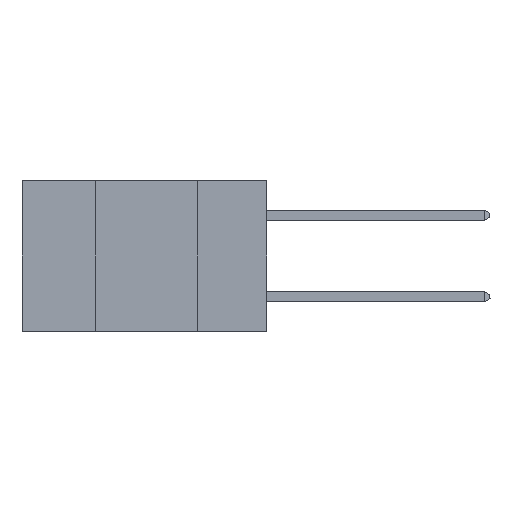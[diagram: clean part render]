
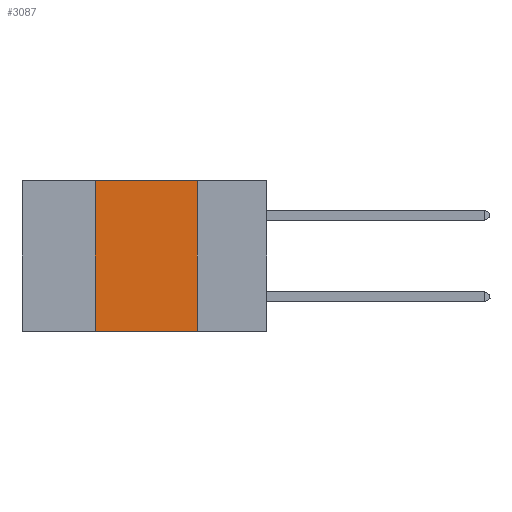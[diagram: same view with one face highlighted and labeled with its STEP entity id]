
A CAD part, left-side view. The second image highlights one B-rep face of the part: STEP entity #3087.
In plain terms, the highlighted planar face has unit normal (-1, 0, 0).
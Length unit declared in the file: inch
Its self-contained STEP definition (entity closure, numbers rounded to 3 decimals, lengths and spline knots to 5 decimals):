
#590 = ORIENTED_EDGE ( 'NONE', *, *, #20053, .F. ) ;
#2403 = VECTOR ( 'NONE', #11665, 39.37008 ) ;
#2624 = VERTEX_POINT ( 'NONE', #2808 ) ;
#2665 = VECTOR ( 'NONE', #20185, 39.37008 ) ;
#2808 = CARTESIAN_POINT ( 'NONE',  ( 0., 0.42, 0. ) ) ;
#3070 = ORIENTED_EDGE ( 'NONE', *, *, #12873, .F. ) ;
#3087 = ADVANCED_FACE ( 'NONE', ( #8059 ), #4212, .F. ) ;
#3782 = DIRECTION ( 'NONE',  ( 0., 0., 1. ) ) ;
#4212 = PLANE ( 'NONE',  #8261 ) ;
#5167 = ORIENTED_EDGE ( 'NONE', *, *, #10167, .T. ) ;
#7063 = CARTESIAN_POINT ( 'NONE',  ( 0., 0.17, 0. ) ) ;
#7428 = DIRECTION ( 'NONE',  ( 1., 0., 0. ) ) ;
#7642 = VECTOR ( 'NONE', #3782, 39.37008 ) ;
#8059 = FACE_OUTER_BOUND ( 'NONE', #15753, .T. ) ;
#8261 = AXIS2_PLACEMENT_3D ( 'NONE', #18558, #7428, #18916 ) ;
#9760 = CARTESIAN_POINT ( 'NONE',  ( 0., 0.17, 0. ) ) ;
#10031 = CARTESIAN_POINT ( 'NONE',  ( 0., 0.6, -0.37 ) ) ;
#10167 = EDGE_CURVE ( 'NONE', #20026, #18764, #10892, .T. ) ;
#10632 = DIRECTION ( 'NONE',  ( 0., 0., -1. ) ) ;
#10892 = LINE ( 'NONE', #10031, #2403 ) ;
#11665 = DIRECTION ( 'NONE',  ( 0., -1., 0. ) ) ;
#11846 = EDGE_CURVE ( 'NONE', #2624, #18517, #12904, .T. ) ;
#12873 = EDGE_CURVE ( 'NONE', #20026, #2624, #14572, .T. ) ;
#12904 = LINE ( 'NONE', #15291, #2665 ) ;
#13332 = CARTESIAN_POINT ( 'NONE',  ( 0., 0.42, 0. ) ) ;
#13747 = CARTESIAN_POINT ( 'NONE',  ( 0., 0.17, -0.37 ) ) ;
#13811 = VECTOR ( 'NONE', #10632, 39.37008 ) ;
#14572 = LINE ( 'NONE', #13332, #7642 ) ;
#15291 = CARTESIAN_POINT ( 'NONE',  ( 0., 0.6, 0. ) ) ;
#15753 = EDGE_LOOP ( 'NONE', ( #590, #19550, #3070, #5167 ) ) ;
#16697 = CARTESIAN_POINT ( 'NONE',  ( 0., 0.42, -0.37 ) ) ;
#18517 = VERTEX_POINT ( 'NONE', #9760 ) ;
#18558 = CARTESIAN_POINT ( 'NONE',  ( 0., 0.6, 0. ) ) ;
#18764 = VERTEX_POINT ( 'NONE', #13747 ) ;
#18916 = DIRECTION ( 'NONE',  ( 0., 0., -1. ) ) ;
#19081 = LINE ( 'NONE', #7063, #13811 ) ;
#19550 = ORIENTED_EDGE ( 'NONE', *, *, #11846, .F. ) ;
#20026 = VERTEX_POINT ( 'NONE', #16697 ) ;
#20053 = EDGE_CURVE ( 'NONE', #18517, #18764, #19081, .T. ) ;
#20185 = DIRECTION ( 'NONE',  ( 0., -1., 0. ) ) ;
